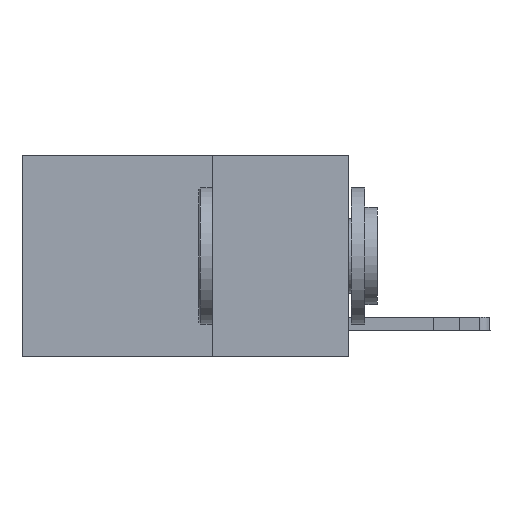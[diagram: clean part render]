
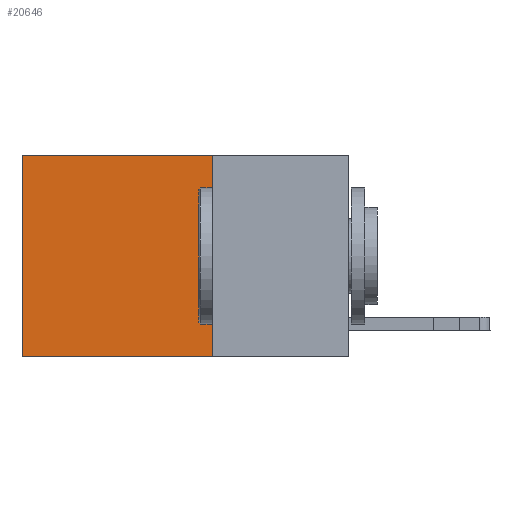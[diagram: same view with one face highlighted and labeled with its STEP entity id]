
A CAD part, left-side view. The second image highlights one B-rep face of the part: STEP entity #20646.
In plain terms, the highlighted planar face has unit normal (-1, 0, 0).
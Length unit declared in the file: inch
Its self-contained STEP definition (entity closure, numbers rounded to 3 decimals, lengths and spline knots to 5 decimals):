
#704 = DIRECTION ( 'NONE',  ( 0., 0., -1. ) ) ;
#2125 = DIRECTION ( 'NONE',  ( 1., 0., 0. ) ) ;
#4588 = VERTEX_POINT ( 'NONE', #15809 ) ;
#4759 = LINE ( 'NONE', #17947, #5298 ) ;
#5295 = ORIENTED_EDGE ( 'NONE', *, *, #5524, .F. ) ;
#5298 = VECTOR ( 'NONE', #16091, 39.37008 ) ;
#5524 = EDGE_CURVE ( 'NONE', #4588, #16122, #15545, .T. ) ;
#5680 = AXIS2_PLACEMENT_3D ( 'NONE', #6455, #2125, #14053 ) ;
#5966 = CARTESIAN_POINT ( 'NONE',  ( 0.2625, 0.6, -0.37 ) ) ;
#6455 = CARTESIAN_POINT ( 'NONE',  ( 0.2625, 0.25, 0. ) ) ;
#6612 = CARTESIAN_POINT ( 'NONE',  ( 0.2625, 0.25, -0.37 ) ) ;
#7487 = LINE ( 'NONE', #16926, #11358 ) ;
#9096 = VECTOR ( 'NONE', #704, 39.37008 ) ;
#10201 = EDGE_LOOP ( 'NONE', ( #12918, #22657, #5295, #19225 ) ) ;
#10915 = CARTESIAN_POINT ( 'NONE',  ( 0.2625, 0.6, 0. ) ) ;
#11218 = EDGE_CURVE ( 'NONE', #16122, #22170, #21703, .T. ) ;
#11358 = VECTOR ( 'NONE', #22765, 39.37008 ) ;
#11603 = PLANE ( 'NONE',  #5680 ) ;
#11952 = EDGE_CURVE ( 'NONE', #19993, #22170, #4759, .T. ) ;
#12918 = ORIENTED_EDGE ( 'NONE', *, *, #11952, .T. ) ;
#14053 = DIRECTION ( 'NONE',  ( 0., 0., -1. ) ) ;
#14209 = DIRECTION ( 'NONE',  ( 0., 1., 0. ) ) ;
#14409 = VECTOR ( 'NONE', #14209, 39.37008 ) ;
#15545 = LINE ( 'NONE', #17518, #9096 ) ;
#15809 = CARTESIAN_POINT ( 'NONE',  ( 0.2625, 0.25, 0. ) ) ;
#16091 = DIRECTION ( 'NONE',  ( 0., 0., -1. ) ) ;
#16122 = VERTEX_POINT ( 'NONE', #20822 ) ;
#16518 = EDGE_CURVE ( 'NONE', #4588, #19993, #7487, .T. ) ;
#16926 = CARTESIAN_POINT ( 'NONE',  ( 0.2625, 0.25, 0. ) ) ;
#17518 = CARTESIAN_POINT ( 'NONE',  ( 0.2625, 0.25, 0. ) ) ;
#17947 = CARTESIAN_POINT ( 'NONE',  ( 0.2625, 0.6, 0. ) ) ;
#19225 = ORIENTED_EDGE ( 'NONE', *, *, #16518, .T. ) ;
#19993 = VERTEX_POINT ( 'NONE', #10915 ) ;
#20646 = ADVANCED_FACE ( 'NONE', ( #23531 ), #11603, .F. ) ;
#20822 = CARTESIAN_POINT ( 'NONE',  ( 0.2625, 0.25, -0.37 ) ) ;
#21703 = LINE ( 'NONE', #6612, #14409 ) ;
#22170 = VERTEX_POINT ( 'NONE', #5966 ) ;
#22657 = ORIENTED_EDGE ( 'NONE', *, *, #11218, .F. ) ;
#22765 = DIRECTION ( 'NONE',  ( 0., 1., 0. ) ) ;
#23531 = FACE_OUTER_BOUND ( 'NONE', #10201, .T. ) ;
